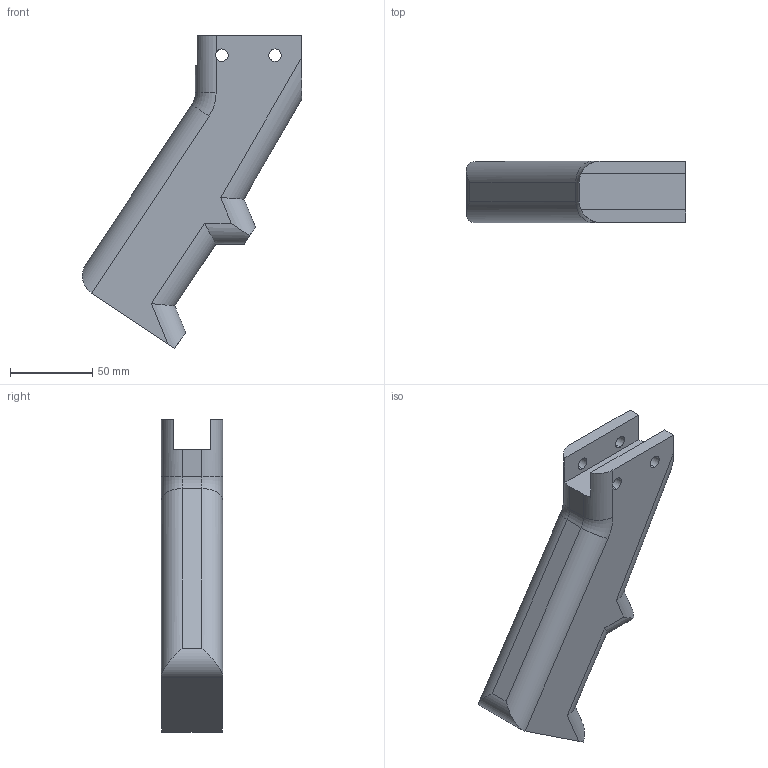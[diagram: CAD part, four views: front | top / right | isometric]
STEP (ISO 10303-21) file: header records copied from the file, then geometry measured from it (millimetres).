
FILE_DESCRIPTION (( 'STEP AP214' ), '1' );
FILE_NAME ('44_grip.STEP', '2013-09-07T19:00:47', ( '' ), ( '' ), 'SwSTEP 2.0', 'SolidWorks 2013', '' );
FILE_SCHEMA (( 'AUTOMOTIVE_DESIGN' ));
Length unit declared in the file: inch
Products named in the file (1): 44_grip
Bounding box: 133.52 x 37.34 x 190.5 mm (x, y, z)
Volume: 390902.9 mm3; surface area: 41667.5 mm2
Topology: 1 solids, 1 shells, 44 faces, 120 edges, 76 vertices
Faces by surface type: cylinder 24, plane 18, torus 2
Entity records: 1448 total; most frequent: CARTESIAN_POINT 319, ORIENTED_EDGE 240, DIRECTION 218, EDGE_CURVE 120, VERTEX_POINT 76, AXIS2_PLACEMENT_3D 75, VECTOR 68, LINE 68
